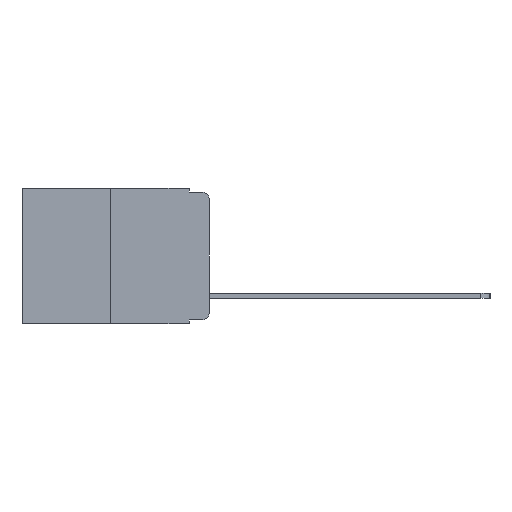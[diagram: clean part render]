
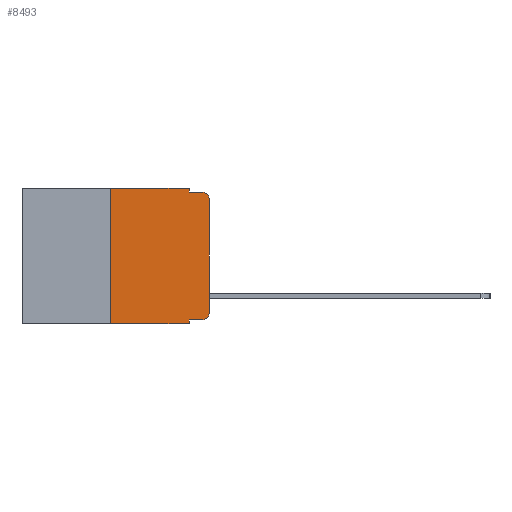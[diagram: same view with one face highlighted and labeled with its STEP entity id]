
A CAD part, left-side view. The second image highlights one B-rep face of the part: STEP entity #8493.
In plain terms, the highlighted planar face has unit normal (-1, 0, 0).
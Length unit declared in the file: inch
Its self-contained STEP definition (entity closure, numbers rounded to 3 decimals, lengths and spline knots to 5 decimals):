
#14 = CARTESIAN_POINT ( 'NONE',  ( 0., 0.051, 0. ) ) ;
#21 = ORIENTED_EDGE ( 'NONE', *, *, #9857, .F. ) ;
#85 = VECTOR ( 'NONE', #840, 39.37008 ) ;
#240 = VERTEX_POINT ( 'NONE', #5393 ) ;
#489 = VECTOR ( 'NONE', #6400, 39.37008 ) ;
#494 = VERTEX_POINT ( 'NONE', #10069 ) ;
#666 = DIRECTION ( 'NONE',  ( -1., 0., 0. ) ) ;
#840 = DIRECTION ( 'NONE',  ( 0., 0., 1. ) ) ;
#947 = CARTESIAN_POINT ( 'NONE',  ( 0., 0.25, 0. ) ) ;
#971 = VECTOR ( 'NONE', #8346, 39.37008 ) ;
#1122 = CARTESIAN_POINT ( 'NONE',  ( 0., 0.051, -0.01 ) ) ;
#1624 = EDGE_LOOP ( 'NONE', ( #10076, #3295, #21, #11202, #8054, #3915, #2244, #7193, #7531, #2515 ) ) ;
#2229 = CARTESIAN_POINT ( 'NONE',  ( 0., 0.473, 0. ) ) ;
#2244 = ORIENTED_EDGE ( 'NONE', *, *, #3137, .T. ) ;
#2515 = ORIENTED_EDGE ( 'NONE', *, *, #10491, .T. ) ;
#2734 = VECTOR ( 'NONE', #5533, 39.37008 ) ;
#2747 = VERTEX_POINT ( 'NONE', #10830 ) ;
#2877 = LINE ( 'NONE', #5574, #9186 ) ;
#2912 = CARTESIAN_POINT ( 'NONE',  ( 0., 0.051, -0.333 ) ) ;
#3023 = LINE ( 'NONE', #14, #2734 ) ;
#3103 = VERTEX_POINT ( 'NONE', #947 ) ;
#3137 = EDGE_CURVE ( 'NONE', #4768, #240, #10453, .T. ) ;
#3183 = AXIS2_PLACEMENT_3D ( 'NONE', #11040, #4185, #8224 ) ;
#3295 = ORIENTED_EDGE ( 'NONE', *, *, #7652, .T. ) ;
#3464 = LINE ( 'NONE', #6723, #971 ) ;
#3682 = VERTEX_POINT ( 'NONE', #5815 ) ;
#3703 = VERTEX_POINT ( 'NONE', #3954 ) ;
#3750 = DIRECTION ( 'NONE',  ( 0., 0., -1. ) ) ;
#3828 = DIRECTION ( 'NONE',  ( 0., 0., -1. ) ) ;
#3830 = VECTOR ( 'NONE', #7381, 39.37008 ) ;
#3915 = ORIENTED_EDGE ( 'NONE', *, *, #7164, .F. ) ;
#3954 = CARTESIAN_POINT ( 'NONE',  ( 0., 0.051, -0.01 ) ) ;
#4185 = DIRECTION ( 'NONE',  ( -1., 0., 0. ) ) ;
#4275 = VERTEX_POINT ( 'NONE', #2912 ) ;
#4736 = CARTESIAN_POINT ( 'NONE',  ( 0., 0.473, -0.343 ) ) ;
#4768 = VERTEX_POINT ( 'NONE', #7060 ) ;
#4793 = DIRECTION ( 'NONE',  ( 0., -1., 0. ) ) ;
#4941 = AXIS2_PLACEMENT_3D ( 'NONE', #2229, #8863, #3750 ) ;
#5017 = CARTESIAN_POINT ( 'NONE',  ( 0., 0., 0. ) ) ;
#5328 = LINE ( 'NONE', #5017, #85 ) ;
#5393 = CARTESIAN_POINT ( 'NONE',  ( 0., 0.051, -0.343 ) ) ;
#5533 = DIRECTION ( 'NONE',  ( 0., 0., -1. ) ) ;
#5574 = CARTESIAN_POINT ( 'NONE',  ( 0., 0.051, 0. ) ) ;
#5778 = VECTOR ( 'NONE', #6647, 39.37008 ) ;
#5815 = CARTESIAN_POINT ( 'NONE',  ( 0., 0.02, -0.01 ) ) ;
#5825 = CARTESIAN_POINT ( 'NONE',  ( 0., 0.473, 0. ) ) ;
#5868 = LINE ( 'NONE', #1122, #3830 ) ;
#5942 = EDGE_CURVE ( 'NONE', #6471, #494, #5328, .T. ) ;
#6021 = VECTOR ( 'NONE', #4793, 39.37008 ) ;
#6034 = CARTESIAN_POINT ( 'NONE',  ( 0., 0.02, -0.333 ) ) ;
#6095 = CARTESIAN_POINT ( 'NONE',  ( 0., 0.02, -0.313 ) ) ;
#6400 = DIRECTION ( 'NONE',  ( 0., -1., 0. ) ) ;
#6471 = VERTEX_POINT ( 'NONE', #7446 ) ;
#6581 = FACE_OUTER_BOUND ( 'NONE', #1624, .T. ) ;
#6647 = DIRECTION ( 'NONE',  ( 0., -1., 0. ) ) ;
#6723 = CARTESIAN_POINT ( 'NONE',  ( 0., 0.25, 0. ) ) ;
#6975 = DIRECTION ( 'NONE',  ( 0., 0., -1. ) ) ;
#7060 = CARTESIAN_POINT ( 'NONE',  ( 0., 0.25, -0.343 ) ) ;
#7164 = EDGE_CURVE ( 'NONE', #4768, #3103, #3464, .T. ) ;
#7193 = ORIENTED_EDGE ( 'NONE', *, *, #8321, .F. ) ;
#7381 = DIRECTION ( 'NONE',  ( 0., -1., 0. ) ) ;
#7426 = VERTEX_POINT ( 'NONE', #6034 ) ;
#7446 = CARTESIAN_POINT ( 'NONE',  ( 0., 0., -0.313 ) ) ;
#7531 = ORIENTED_EDGE ( 'NONE', *, *, #8301, .T. ) ;
#7652 = EDGE_CURVE ( 'NONE', #494, #3682, #7787, .T. ) ;
#7787 = CIRCLE ( 'NONE', #3183, 0.02 ) ;
#7900 = LINE ( 'NONE', #8724, #489 ) ;
#8054 = ORIENTED_EDGE ( 'NONE', *, *, #8474, .F. ) ;
#8224 = DIRECTION ( 'NONE',  ( 0., 0., -1. ) ) ;
#8301 = EDGE_CURVE ( 'NONE', #4275, #7426, #7900, .T. ) ;
#8321 = EDGE_CURVE ( 'NONE', #4275, #240, #3023, .T. ) ;
#8346 = DIRECTION ( 'NONE',  ( 0., 0., 1. ) ) ;
#8434 = CIRCLE ( 'NONE', #10174, 0.02 ) ;
#8474 = EDGE_CURVE ( 'NONE', #3103, #2747, #10201, .T. ) ;
#8493 = ADVANCED_FACE ( 'NONE', ( #6581 ), #9202, .F. ) ;
#8724 = CARTESIAN_POINT ( 'NONE',  ( 0., 0.051, -0.333 ) ) ;
#8863 = DIRECTION ( 'NONE',  ( 1., 0., 0. ) ) ;
#9186 = VECTOR ( 'NONE', #3828, 39.37008 ) ;
#9202 = PLANE ( 'NONE',  #4941 ) ;
#9857 = EDGE_CURVE ( 'NONE', #3703, #3682, #5868, .T. ) ;
#10069 = CARTESIAN_POINT ( 'NONE',  ( 0., 0., -0.03 ) ) ;
#10076 = ORIENTED_EDGE ( 'NONE', *, *, #5942, .T. ) ;
#10174 = AXIS2_PLACEMENT_3D ( 'NONE', #6095, #666, #6975 ) ;
#10201 = LINE ( 'NONE', #5825, #5778 ) ;
#10453 = LINE ( 'NONE', #4736, #6021 ) ;
#10491 = EDGE_CURVE ( 'NONE', #7426, #6471, #8434, .T. ) ;
#10830 = CARTESIAN_POINT ( 'NONE',  ( 0., 0.051, 0. ) ) ;
#11040 = CARTESIAN_POINT ( 'NONE',  ( 0., 0.02, -0.03 ) ) ;
#11202 = ORIENTED_EDGE ( 'NONE', *, *, #11245, .F. ) ;
#11245 = EDGE_CURVE ( 'NONE', #2747, #3703, #2877, .T. ) ;
